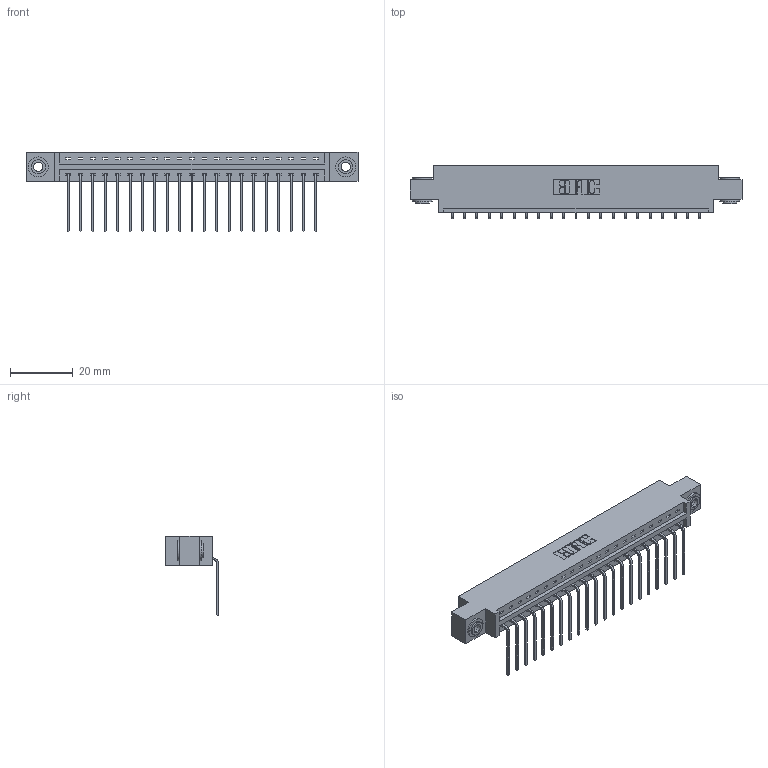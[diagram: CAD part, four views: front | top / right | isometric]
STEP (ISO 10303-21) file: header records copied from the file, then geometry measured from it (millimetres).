
FILE_DESCRIPTION (( 'STEP AP203' ), '1' );
FILE_NAME ('387-021-559-603.STEP', '2018-09-14T02:47:26', ( '' ), ( '' ), 'SwSTEP 2.0', 'SolidWorks 2016', '' );
FILE_SCHEMA (( 'CONFIG_CONTROL_DESIGN' ));
Length unit declared in the file: inch
Products named in the file (4): 345-250-002_345-250-002-102; 387-021-559-603; 337 Part_0.170 Offset - 0.156 Dia-TH; 345-292-001_558 559 Tail - 1
Assembly tree (24 placements, depth 2):
  387-021-559-603
    337 Part_0.170 Offset - 0.156 Dia-TH
    345-292-001_558 559 Tail - 1  x21
    345-250-002_345-250-002-102  x2
Bounding box: 106.22 x 17.09 x 25.53 mm (x, y, z)
Volume: 10749.1 mm3; surface area: 11750.1 mm2
Topology: 24 solids, 24 shells, 1500 faces, 4473 edges, 2950 vertices
Faces by surface type: plane 1092, cylinder 400, cone 8
Entity records: 19192 total; most frequent: CARTESIAN_POINT 3320, ORIENTED_EDGE 3270, DIRECTION 2871, EDGE_CURVE 1635, VECTOR 1483, LINE 1483, VERTEX_POINT 1086, AXIS2_PLACEMENT_3D 694
